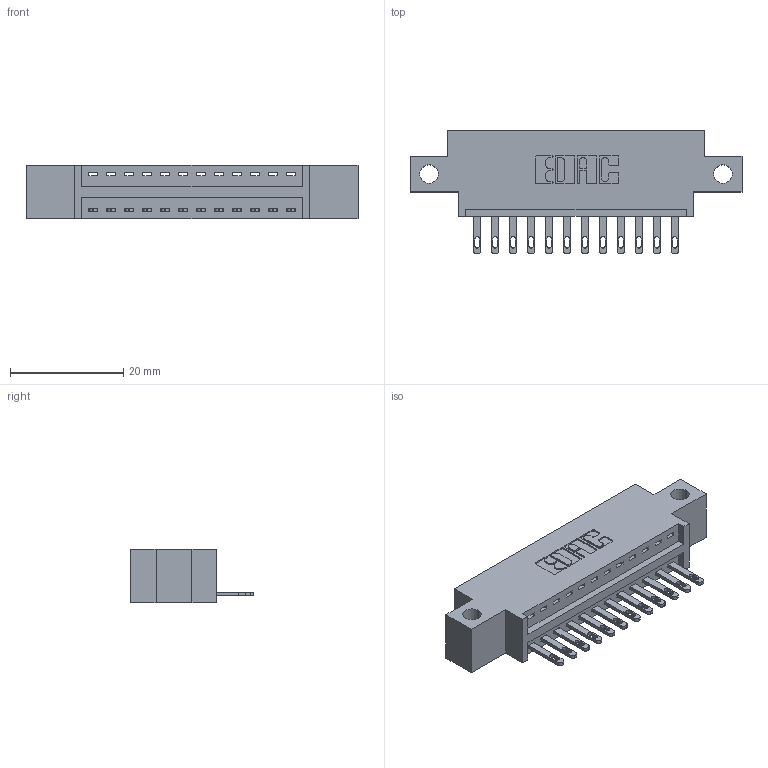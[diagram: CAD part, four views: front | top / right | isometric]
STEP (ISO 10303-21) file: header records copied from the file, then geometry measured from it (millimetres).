
FILE_DESCRIPTION (( 'STEP AP203' ), '1' );
FILE_NAME ('346-012-500-612.STEP', '2018-08-19T21:39:31', ( '' ), ( '' ), 'SwSTEP 2.0', 'SolidWorks 2016', '' );
FILE_SCHEMA (( 'CONFIG_CONTROL_DESIGN' ));
Length unit declared in the file: inch
Products named in the file (3): 346 Part_0.170 Offset - Side Mount; 345-292-001_345-293-100; 346-012-500-612
Assembly tree (13 placements, depth 2):
  346-012-500-612
    346 Part_0.170 Offset - Side Mount
    345-292-001_345-293-100  x12
Bounding box: 58.67 x 21.84 x 9.4 mm (x, y, z)
Volume: 5175.2 mm3; surface area: 6187.2 mm2
Topology: 13 solids, 13 shells, 774 faces, 2357 edges, 1570 vertices
Faces by surface type: plane 488, cylinder 286
Entity records: 11551 total; most frequent: CARTESIAN_POINT 1996, ORIENTED_EDGE 1942, DIRECTION 1799, EDGE_CURVE 971, LINE 787, VECTOR 787, VERTEX_POINT 646, AXIS2_PLACEMENT_3D 506
